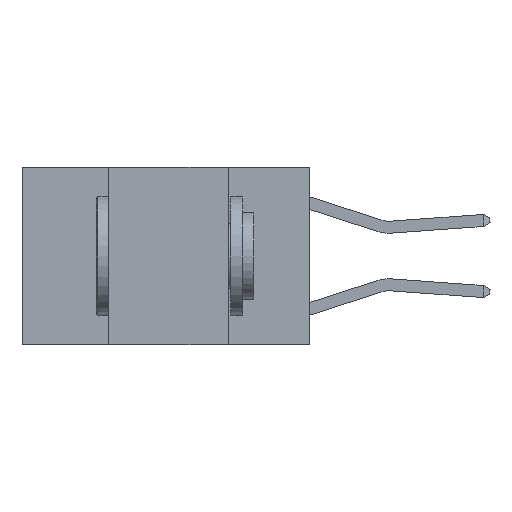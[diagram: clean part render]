
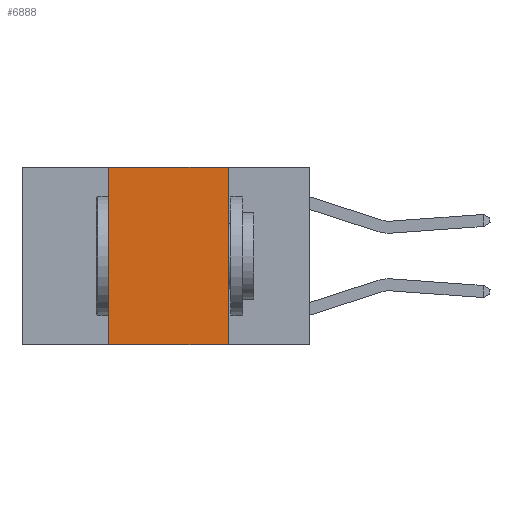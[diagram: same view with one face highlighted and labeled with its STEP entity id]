
A CAD part, left-side view. The second image highlights one B-rep face of the part: STEP entity #6888.
In plain terms, the highlighted planar face has unit normal (-1, 0, 0).
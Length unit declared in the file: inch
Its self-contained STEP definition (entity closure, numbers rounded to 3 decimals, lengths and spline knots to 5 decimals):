
#347 = DIRECTION ( 'NONE',  ( 1., 0., 0. ) ) ;
#1288 = DIRECTION ( 'NONE',  ( 0., 0., -1. ) ) ;
#1897 = VERTEX_POINT ( 'NONE', #14162 ) ;
#2407 = ORIENTED_EDGE ( 'NONE', *, *, #12671, .F. ) ;
#2614 = LINE ( 'NONE', #6020, #8454 ) ;
#2955 = EDGE_LOOP ( 'NONE', ( #9995, #2407, #7242, #5432 ) ) ;
#4416 = VECTOR ( 'NONE', #10152, 39.37008 ) ;
#4488 = CARTESIAN_POINT ( 'NONE',  ( 0., 0.6, -0.37 ) ) ;
#4732 = CARTESIAN_POINT ( 'NONE',  ( 0., 0.17, 0. ) ) ;
#4957 = LINE ( 'NONE', #11936, #9699 ) ;
#5432 = ORIENTED_EDGE ( 'NONE', *, *, #8758, .T. ) ;
#5908 = DIRECTION ( 'NONE',  ( 0., -1., 0. ) ) ;
#6020 = CARTESIAN_POINT ( 'NONE',  ( 0., 0.17, 0. ) ) ;
#6888 = ADVANCED_FACE ( 'NONE', ( #7618 ), #12335, .F. ) ;
#7242 = ORIENTED_EDGE ( 'NONE', *, *, #14872, .F. ) ;
#7274 = DIRECTION ( 'NONE',  ( 0., 0., 1. ) ) ;
#7618 = FACE_OUTER_BOUND ( 'NONE', #2955, .T. ) ;
#7762 = LINE ( 'NONE', #4488, #4416 ) ;
#8204 = CARTESIAN_POINT ( 'NONE',  ( 0., 0.17, -0.37 ) ) ;
#8209 = EDGE_CURVE ( 'NONE', #10437, #9463, #2614, .T. ) ;
#8229 = VERTEX_POINT ( 'NONE', #10806 ) ;
#8454 = VECTOR ( 'NONE', #1288, 39.37008 ) ;
#8758 = EDGE_CURVE ( 'NONE', #8229, #9463, #7762, .T. ) ;
#9463 = VERTEX_POINT ( 'NONE', #8204 ) ;
#9699 = VECTOR ( 'NONE', #5908, 39.37008 ) ;
#9722 = VECTOR ( 'NONE', #7274, 39.37008 ) ;
#9871 = CARTESIAN_POINT ( 'NONE',  ( 0., 0.6, 0. ) ) ;
#9995 = ORIENTED_EDGE ( 'NONE', *, *, #8209, .F. ) ;
#10152 = DIRECTION ( 'NONE',  ( 0., -1., 0. ) ) ;
#10437 = VERTEX_POINT ( 'NONE', #4732 ) ;
#10806 = CARTESIAN_POINT ( 'NONE',  ( 0., 0.42, -0.37 ) ) ;
#11936 = CARTESIAN_POINT ( 'NONE',  ( 0., 0.6, 0. ) ) ;
#12102 = DIRECTION ( 'NONE',  ( 0., 0., -1. ) ) ;
#12335 = PLANE ( 'NONE',  #13805 ) ;
#12671 = EDGE_CURVE ( 'NONE', #1897, #10437, #4957, .T. ) ;
#13219 = LINE ( 'NONE', #15212, #9722 ) ;
#13805 = AXIS2_PLACEMENT_3D ( 'NONE', #9871, #347, #12102 ) ;
#14162 = CARTESIAN_POINT ( 'NONE',  ( 0., 0.42, 0. ) ) ;
#14872 = EDGE_CURVE ( 'NONE', #8229, #1897, #13219, .T. ) ;
#15212 = CARTESIAN_POINT ( 'NONE',  ( 0., 0.42, 0. ) ) ;
